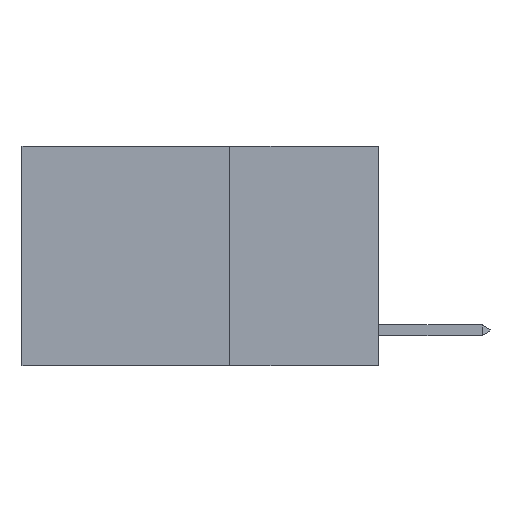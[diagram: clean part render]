
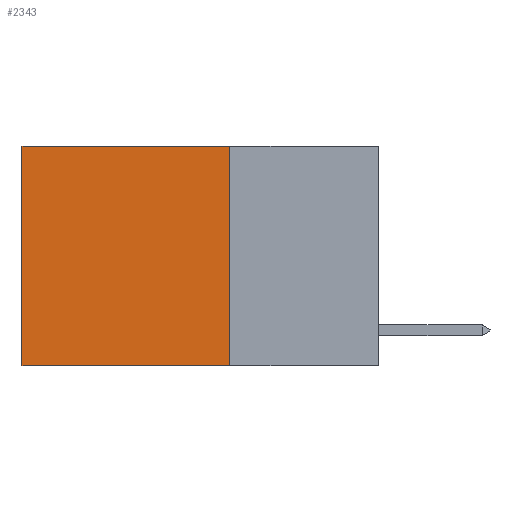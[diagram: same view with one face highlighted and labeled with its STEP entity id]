
A CAD part, left-side view. The second image highlights one B-rep face of the part: STEP entity #2343.
In plain terms, the highlighted planar face has unit normal (-1, 0, 0).
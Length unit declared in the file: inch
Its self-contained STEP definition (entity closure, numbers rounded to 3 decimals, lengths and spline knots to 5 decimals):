
#489 = DIRECTION ( 'NONE',  ( 0., 1., 0. ) ) ;
#1080 = DIRECTION ( 'NONE',  ( 0., 1., 0. ) ) ;
#2239 = LINE ( 'NONE', #5424, #2347 ) ;
#2343 = ADVANCED_FACE ( 'NONE', ( #15287 ), #7657, .F. ) ;
#2347 = VECTOR ( 'NONE', #1080, 39.37008 ) ;
#2480 = ORIENTED_EDGE ( 'NONE', *, *, #15671, .T. ) ;
#3393 = DIRECTION ( 'NONE',  ( 0., 0., -1. ) ) ;
#3589 = CARTESIAN_POINT ( 'NONE',  ( 0.2625, 0.25, -0.37 ) ) ;
#3863 = EDGE_CURVE ( 'NONE', #5631, #16812, #2239, .T. ) ;
#4139 = CARTESIAN_POINT ( 'NONE',  ( 0.2625, 0.25, -0.37 ) ) ;
#5276 = EDGE_CURVE ( 'NONE', #16670, #13338, #12384, .T. ) ;
#5424 = CARTESIAN_POINT ( 'NONE',  ( 0.2625, 0.25, 0. ) ) ;
#5631 = VERTEX_POINT ( 'NONE', #14383 ) ;
#5671 = VECTOR ( 'NONE', #17780, 39.37008 ) ;
#5731 = LINE ( 'NONE', #17534, #9348 ) ;
#7657 = PLANE ( 'NONE',  #13089 ) ;
#7681 = ORIENTED_EDGE ( 'NONE', *, *, #5276, .F. ) ;
#8839 = ORIENTED_EDGE ( 'NONE', *, *, #3863, .T. ) ;
#9065 = LINE ( 'NONE', #16313, #5671 ) ;
#9109 = CARTESIAN_POINT ( 'NONE',  ( 0.2625, 0.25, 0. ) ) ;
#9348 = VECTOR ( 'NONE', #17439, 39.37008 ) ;
#10417 = VECTOR ( 'NONE', #489, 39.37008 ) ;
#10742 = DIRECTION ( 'NONE',  ( 1., 0., 0. ) ) ;
#12038 = ORIENTED_EDGE ( 'NONE', *, *, #16744, .F. ) ;
#12384 = LINE ( 'NONE', #3589, #10417 ) ;
#13089 = AXIS2_PLACEMENT_3D ( 'NONE', #9109, #10742, #3393 ) ;
#13338 = VERTEX_POINT ( 'NONE', #17934 ) ;
#13750 = EDGE_LOOP ( 'NONE', ( #2480, #7681, #12038, #8839 ) ) ;
#14383 = CARTESIAN_POINT ( 'NONE',  ( 0.2625, 0.25, 0. ) ) ;
#14590 = CARTESIAN_POINT ( 'NONE',  ( 0.2625, 0.6, 0. ) ) ;
#15287 = FACE_OUTER_BOUND ( 'NONE', #13750, .T. ) ;
#15671 = EDGE_CURVE ( 'NONE', #16812, #13338, #5731, .T. ) ;
#16313 = CARTESIAN_POINT ( 'NONE',  ( 0.2625, 0.25, 0. ) ) ;
#16670 = VERTEX_POINT ( 'NONE', #4139 ) ;
#16744 = EDGE_CURVE ( 'NONE', #5631, #16670, #9065, .T. ) ;
#16812 = VERTEX_POINT ( 'NONE', #14590 ) ;
#17439 = DIRECTION ( 'NONE',  ( 0., 0., -1. ) ) ;
#17534 = CARTESIAN_POINT ( 'NONE',  ( 0.2625, 0.6, 0. ) ) ;
#17780 = DIRECTION ( 'NONE',  ( 0., 0., -1. ) ) ;
#17934 = CARTESIAN_POINT ( 'NONE',  ( 0.2625, 0.6, -0.37 ) ) ;
